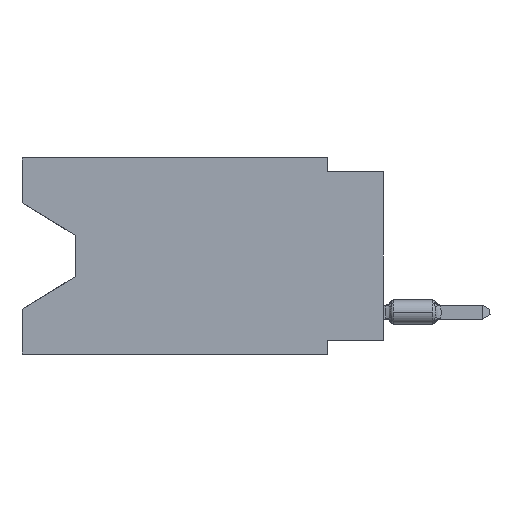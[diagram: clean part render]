
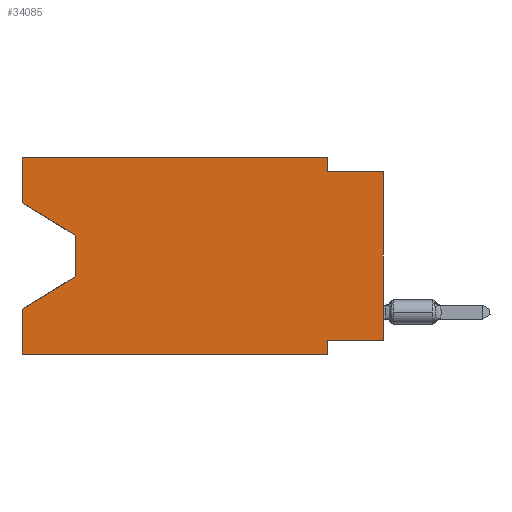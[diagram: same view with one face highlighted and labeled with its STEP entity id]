
A CAD part, left-side view. The second image highlights one B-rep face of the part: STEP entity #34085.
In plain terms, the highlighted planar face has unit normal (-1, 0, 0).
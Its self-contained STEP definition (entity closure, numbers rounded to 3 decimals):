
#907 = CARTESIAN_POINT ( 'NONE',  ( 0., 13.97, -5.385 ) ) ;
#1169 = LINE ( 'NONE', #54974, #34024 ) ;
#1635 = ORIENTED_EDGE ( 'NONE', *, *, #47873, .F. ) ;
#1802 = ORIENTED_EDGE ( 'NONE', *, *, #4150, .T. ) ;
#2307 = DIRECTION ( 'NONE',  ( 0., 0., -1. ) ) ;
#3505 = VERTEX_POINT ( 'NONE', #23601 ) ;
#3805 = VECTOR ( 'NONE', #10533, 1000. ) ;
#4024 = VECTOR ( 'NONE', #2307, 1000. ) ;
#4150 = EDGE_CURVE ( 'NONE', #11860, #6070, #54608, .T. ) ;
#4457 = PLANE ( 'NONE',  #30201 ) ;
#4805 = LINE ( 'NONE', #41664, #30899 ) ;
#5951 = VECTOR ( 'NONE', #36488, 1000. ) ;
#6070 = VERTEX_POINT ( 'NONE', #51260 ) ;
#7271 = ORIENTED_EDGE ( 'NONE', *, *, #34198, .T. ) ;
#7649 = EDGE_CURVE ( 'NONE', #51144, #26918, #37803, .T. ) ;
#8013 = DIRECTION ( 'NONE',  ( 0., -1., 0. ) ) ;
#8631 = CARTESIAN_POINT ( 'NONE',  ( 0., 16.383, 0. ) ) ;
#8714 = EDGE_CURVE ( 'NONE', #18766, #57825, #4805, .T. ) ;
#10469 = CARTESIAN_POINT ( 'NONE',  ( 0., 16.383, -6.852 ) ) ;
#10533 = DIRECTION ( 'NONE',  ( 0., 0., -1. ) ) ;
#11392 = VERTEX_POINT ( 'NONE', #53499 ) ;
#11494 = VECTOR ( 'NONE', #45168, 1000. ) ;
#11860 = VERTEX_POINT ( 'NONE', #58469 ) ;
#12373 = CARTESIAN_POINT ( 'NONE',  ( 0., 16.383, 0. ) ) ;
#12559 = CARTESIAN_POINT ( 'NONE',  ( 0., 0., -8.255 ) ) ;
#13096 = FACE_OUTER_BOUND ( 'NONE', #29222, .T. ) ;
#13281 = DIRECTION ( 'NONE',  ( 0., 0., 1. ) ) ;
#13464 = VECTOR ( 'NONE', #43905, 1000. ) ;
#13929 = LINE ( 'NONE', #27885, #11494 ) ;
#14257 = DIRECTION ( 'NONE',  ( 0., -1., 0. ) ) ;
#15633 = EDGE_CURVE ( 'NONE', #3505, #42745, #37594, .T. ) ;
#18606 = CARTESIAN_POINT ( 'NONE',  ( 0., 0., 0. ) ) ;
#18766 = VERTEX_POINT ( 'NONE', #38522 ) ;
#22290 = ORIENTED_EDGE ( 'NONE', *, *, #58668, .F. ) ;
#23574 = CARTESIAN_POINT ( 'NONE',  ( 0., 16.383, 0. ) ) ;
#23601 = CARTESIAN_POINT ( 'NONE',  ( 0., 2.54, -8.255 ) ) ;
#25970 = CARTESIAN_POINT ( 'NONE',  ( 0., 0., -0.635 ) ) ;
#26296 = ORIENTED_EDGE ( 'NONE', *, *, #7649, .F. ) ;
#26780 = CARTESIAN_POINT ( 'NONE',  ( 0., 2.54, 0. ) ) ;
#26918 = VERTEX_POINT ( 'NONE', #26780 ) ;
#27885 = CARTESIAN_POINT ( 'NONE',  ( 0., 16.383, -2.038 ) ) ;
#29222 = EDGE_LOOP ( 'NONE', ( #57502, #1802, #46306, #51717, #7271, #54986, #40364, #49267, #30291, #1635, #26296, #22290 ) ) ;
#29638 = CARTESIAN_POINT ( 'NONE',  ( 0., 16.383, 0. ) ) ;
#30201 = AXIS2_PLACEMENT_3D ( 'NONE', #8631, #54398, #54117 ) ;
#30291 = ORIENTED_EDGE ( 'NONE', *, *, #8714, .F. ) ;
#30701 = DIRECTION ( 'NONE',  ( 0., 1., 0. ) ) ;
#30899 = VECTOR ( 'NONE', #46118, 1000. ) ;
#33316 = VECTOR ( 'NONE', #54793, 1000. ) ;
#34024 = VECTOR ( 'NONE', #14257, 1000. ) ;
#34085 = ADVANCED_FACE ( 'NONE', ( #13096 ), #4457, .F. ) ;
#34198 = EDGE_CURVE ( 'NONE', #42000, #42745, #1169, .T. ) ;
#35287 = EDGE_CURVE ( 'NONE', #11392, #3505, #53292, .T. ) ;
#36387 = CARTESIAN_POINT ( 'NONE',  ( 0., 16.383, -2.038 ) ) ;
#36488 = DIRECTION ( 'NONE',  ( 0., 0., -1. ) ) ;
#37496 = LINE ( 'NONE', #907, #58181 ) ;
#37594 = LINE ( 'NONE', #50667, #3805 ) ;
#37803 = LINE ( 'NONE', #52335, #53606 ) ;
#38522 = CARTESIAN_POINT ( 'NONE',  ( 0., 2.54, -0.635 ) ) ;
#39150 = LINE ( 'NONE', #29638, #13464 ) ;
#40364 = ORIENTED_EDGE ( 'NONE', *, *, #35287, .F. ) ;
#41106 = VERTEX_POINT ( 'NONE', #36387 ) ;
#41664 = CARTESIAN_POINT ( 'NONE',  ( 0., 0., -0.635 ) ) ;
#42000 = VERTEX_POINT ( 'NONE', #42715 ) ;
#42715 = CARTESIAN_POINT ( 'NONE',  ( 0., 16.383, -8.89 ) ) ;
#42745 = VERTEX_POINT ( 'NONE', #54638 ) ;
#43492 = EDGE_CURVE ( 'NONE', #6070, #56002, #37496, .T. ) ;
#43905 = DIRECTION ( 'NONE',  ( 0., 0., 1. ) ) ;
#45123 = VECTOR ( 'NONE', #30701, 1000. ) ;
#45168 = DIRECTION ( 'NONE',  ( 0., -0.855, -0.519 ) ) ;
#46118 = DIRECTION ( 'NONE',  ( 0., -1., 0. ) ) ;
#46181 = LINE ( 'NONE', #23574, #33316 ) ;
#46306 = ORIENTED_EDGE ( 'NONE', *, *, #43492, .T. ) ;
#47807 = LINE ( 'NONE', #56701, #4024 ) ;
#47873 = EDGE_CURVE ( 'NONE', #26918, #18766, #47807, .T. ) ;
#48182 = EDGE_CURVE ( 'NONE', #41106, #11860, #13929, .T. ) ;
#48575 = EDGE_CURVE ( 'NONE', #11392, #57825, #50430, .T. ) ;
#49267 = ORIENTED_EDGE ( 'NONE', *, *, #48575, .T. ) ;
#50430 = LINE ( 'NONE', #18606, #58635 ) ;
#50667 = CARTESIAN_POINT ( 'NONE',  ( 0., 2.54, -8.89 ) ) ;
#51079 = EDGE_CURVE ( 'NONE', #42000, #56002, #39150, .T. ) ;
#51144 = VERTEX_POINT ( 'NONE', #12373 ) ;
#51260 = CARTESIAN_POINT ( 'NONE',  ( 0., 13.97, -5.385 ) ) ;
#51717 = ORIENTED_EDGE ( 'NONE', *, *, #51079, .F. ) ;
#52335 = CARTESIAN_POINT ( 'NONE',  ( 0., 16.383, 0. ) ) ;
#53292 = LINE ( 'NONE', #12559, #45123 ) ;
#53499 = CARTESIAN_POINT ( 'NONE',  ( 0., 0., -8.255 ) ) ;
#53606 = VECTOR ( 'NONE', #8013, 1000. ) ;
#54117 = DIRECTION ( 'NONE',  ( 0., 0., -1. ) ) ;
#54398 = DIRECTION ( 'NONE',  ( 1., 0., 0. ) ) ;
#54608 = LINE ( 'NONE', #58198, #5951 ) ;
#54638 = CARTESIAN_POINT ( 'NONE',  ( 0., 2.54, -8.89 ) ) ;
#54793 = DIRECTION ( 'NONE',  ( 0., 0., 1. ) ) ;
#54974 = CARTESIAN_POINT ( 'NONE',  ( 0., 16.383, -8.89 ) ) ;
#54986 = ORIENTED_EDGE ( 'NONE', *, *, #15633, .F. ) ;
#55613 = DIRECTION ( 'NONE',  ( 0., 0.855, -0.519 ) ) ;
#56002 = VERTEX_POINT ( 'NONE', #10469 ) ;
#56701 = CARTESIAN_POINT ( 'NONE',  ( 0., 2.54, 0. ) ) ;
#57502 = ORIENTED_EDGE ( 'NONE', *, *, #48182, .T. ) ;
#57825 = VERTEX_POINT ( 'NONE', #25970 ) ;
#58181 = VECTOR ( 'NONE', #55613, 1000. ) ;
#58198 = CARTESIAN_POINT ( 'NONE',  ( 0., 13.97, -3.505 ) ) ;
#58469 = CARTESIAN_POINT ( 'NONE',  ( 0., 13.97, -3.505 ) ) ;
#58635 = VECTOR ( 'NONE', #13281, 1000. ) ;
#58668 = EDGE_CURVE ( 'NONE', #41106, #51144, #46181, .T. ) ;
